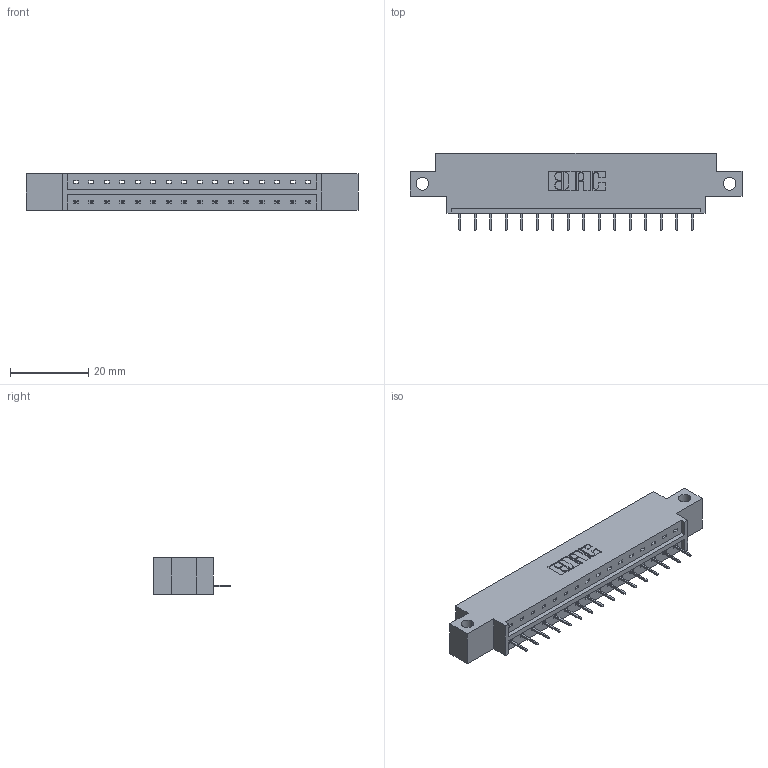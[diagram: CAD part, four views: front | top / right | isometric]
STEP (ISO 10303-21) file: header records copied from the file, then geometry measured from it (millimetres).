
FILE_DESCRIPTION (( 'STEP AP203' ), '1' );
FILE_NAME ('333-016-524-612.STEP', '2018-08-01T11:42:37', ( '' ), ( '' ), 'SwSTEP 2.0', 'SolidWorks 2016', '' );
FILE_SCHEMA (( 'CONFIG_CONTROL_DESIGN' ));
Length unit declared in the file: inch
Products named in the file (3): 345-292-001_345-293-124; 333-016-524-612; 333 Part_Offset - Side
Assembly tree (17 placements, depth 2):
  333-016-524-612
    333 Part_Offset - Side
    345-292-001_345-293-124  x16
Bounding box: 84.94 x 19.69 x 9.4 mm (x, y, z)
Volume: 7945.2 mm3; surface area: 8252 mm2
Topology: 17 solids, 17 shells, 1110 faces, 3203 edges, 2070 vertices
Faces by surface type: plane 842, cylinder 268
Entity records: 13353 total; most frequent: CARTESIAN_POINT 2314, ORIENTED_EDGE 2266, DIRECTION 2005, EDGE_CURVE 1133, LINE 1009, VECTOR 1009, VERTEX_POINT 750, AXIS2_PLACEMENT_3D 498
